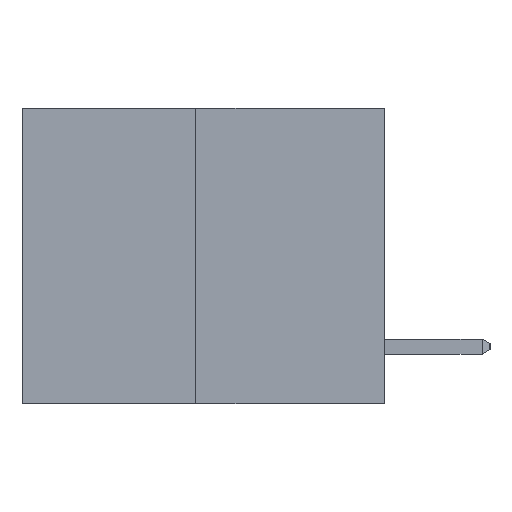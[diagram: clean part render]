
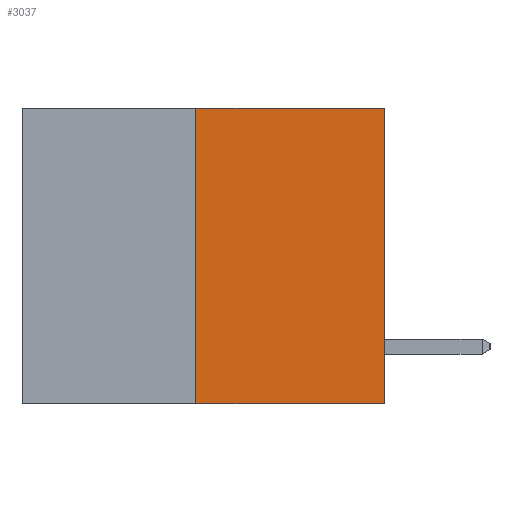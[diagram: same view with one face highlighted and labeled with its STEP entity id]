
A CAD part, left-side view. The second image highlights one B-rep face of the part: STEP entity #3037.
In plain terms, the highlighted planar face has unit normal (-1, 0, 0).
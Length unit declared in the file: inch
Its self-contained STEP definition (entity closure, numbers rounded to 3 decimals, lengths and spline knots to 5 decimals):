
#498 = VERTEX_POINT ( 'NONE', #21121 ) ;
#1191 = VERTEX_POINT ( 'NONE', #15935 ) ;
#1587 = CARTESIAN_POINT ( 'NONE',  ( 0., 0., 0. ) ) ;
#2558 = CARTESIAN_POINT ( 'NONE',  ( 0., 0.6, -0.49 ) ) ;
#2766 = VECTOR ( 'NONE', #4794, 39.37008 ) ;
#3037 = ADVANCED_FACE ( 'NONE', ( #11098 ), #19346, .F. ) ;
#3591 = EDGE_CURVE ( 'NONE', #498, #1191, #6673, .T. ) ;
#3808 = VECTOR ( 'NONE', #17815, 39.37008 ) ;
#4138 = DIRECTION ( 'NONE',  ( 1., 0., 0. ) ) ;
#4274 = DIRECTION ( 'NONE',  ( 0., 0., -1. ) ) ;
#4794 = DIRECTION ( 'NONE',  ( 0., -1., 0. ) ) ;
#5193 = VERTEX_POINT ( 'NONE', #12973 ) ;
#5830 = ORIENTED_EDGE ( 'NONE', *, *, #18541, .F. ) ;
#6007 = ORIENTED_EDGE ( 'NONE', *, *, #13888, .T. ) ;
#6235 = ORIENTED_EDGE ( 'NONE', *, *, #3591, .F. ) ;
#6651 = LINE ( 'NONE', #22056, #10636 ) ;
#6673 = LINE ( 'NONE', #16609, #16235 ) ;
#9449 = DIRECTION ( 'NONE',  ( 0., 0., 1. ) ) ;
#10266 = EDGE_LOOP ( 'NONE', ( #6235, #6007, #15888, #5830 ) ) ;
#10636 = VECTOR ( 'NONE', #15086, 39.37008 ) ;
#11098 = FACE_OUTER_BOUND ( 'NONE', #10266, .T. ) ;
#11253 = VERTEX_POINT ( 'NONE', #1587 ) ;
#12973 = CARTESIAN_POINT ( 'NONE',  ( 0., 0., -0.49 ) ) ;
#13888 = EDGE_CURVE ( 'NONE', #498, #5193, #13935, .T. ) ;
#13935 = LINE ( 'NONE', #2558, #3808 ) ;
#14471 = CARTESIAN_POINT ( 'NONE',  ( 0., 0.6, 0. ) ) ;
#15086 = DIRECTION ( 'NONE',  ( 0., 0., 1. ) ) ;
#15878 = EDGE_CURVE ( 'NONE', #5193, #11253, #6651, .T. ) ;
#15888 = ORIENTED_EDGE ( 'NONE', *, *, #15878, .T. ) ;
#15935 = CARTESIAN_POINT ( 'NONE',  ( 0., 0.312, 0. ) ) ;
#16059 = AXIS2_PLACEMENT_3D ( 'NONE', #14471, #4138, #4274 ) ;
#16235 = VECTOR ( 'NONE', #9449, 39.37008 ) ;
#16609 = CARTESIAN_POINT ( 'NONE',  ( 0., 0.312, -0.49 ) ) ;
#17391 = LINE ( 'NONE', #20226, #2766 ) ;
#17815 = DIRECTION ( 'NONE',  ( 0., -1., 0. ) ) ;
#18541 = EDGE_CURVE ( 'NONE', #1191, #11253, #17391, .T. ) ;
#19346 = PLANE ( 'NONE',  #16059 ) ;
#20226 = CARTESIAN_POINT ( 'NONE',  ( 0., 0.6, 0. ) ) ;
#21121 = CARTESIAN_POINT ( 'NONE',  ( 0., 0.312, -0.49 ) ) ;
#22056 = CARTESIAN_POINT ( 'NONE',  ( 0., 0., 0. ) ) ;
